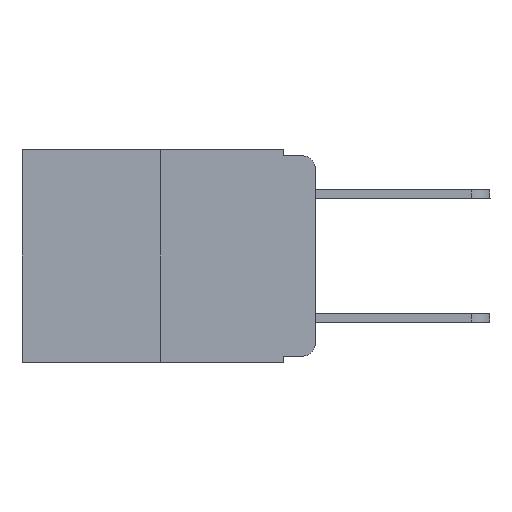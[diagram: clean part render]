
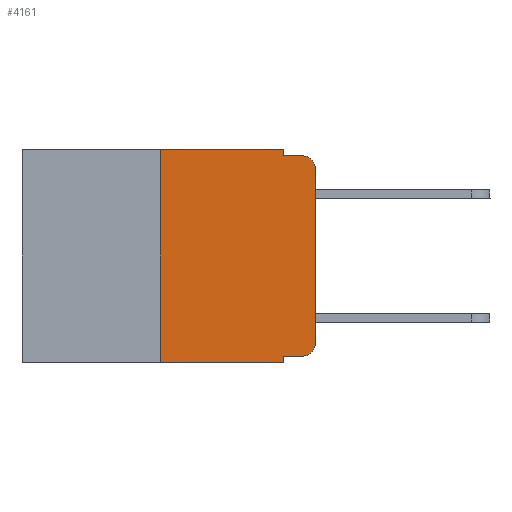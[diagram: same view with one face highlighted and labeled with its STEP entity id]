
A CAD part, left-side view. The second image highlights one B-rep face of the part: STEP entity #4161.
In plain terms, the highlighted planar face has unit normal (-1, 0, 0).
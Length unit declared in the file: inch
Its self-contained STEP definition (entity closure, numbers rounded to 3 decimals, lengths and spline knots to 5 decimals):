
#337 = EDGE_CURVE ( 'NONE', #19525, #14677, #18125, .T. ) ;
#1096 = DIRECTION ( 'NONE',  ( 0., 0., 1. ) ) ;
#1209 = EDGE_CURVE ( 'NONE', #7243, #7101, #4315, .T. ) ;
#1236 = CARTESIAN_POINT ( 'NONE',  ( 0., 0., -0.313 ) ) ;
#1493 = CARTESIAN_POINT ( 'NONE',  ( 0., 0.25, 0. ) ) ;
#1759 = VECTOR ( 'NONE', #14645, 39.37008 ) ;
#1848 = CARTESIAN_POINT ( 'NONE',  ( 0., 0.02, -0.313 ) ) ;
#2387 = CARTESIAN_POINT ( 'NONE',  ( 0., 0.051, -0.343 ) ) ;
#2466 = VECTOR ( 'NONE', #3647, 39.37008 ) ;
#2527 = EDGE_CURVE ( 'NONE', #3661, #4597, #5722, .T. ) ;
#2531 = CARTESIAN_POINT ( 'NONE',  ( 0., 0.25, -0.343 ) ) ;
#2651 = AXIS2_PLACEMENT_3D ( 'NONE', #13378, #22353, #20773 ) ;
#2685 = ORIENTED_EDGE ( 'NONE', *, *, #13599, .T. ) ;
#2820 = EDGE_CURVE ( 'NONE', #5294, #3661, #14529, .T. ) ;
#2821 = LINE ( 'NONE', #6984, #9242 ) ;
#3045 = VECTOR ( 'NONE', #20054, 39.37008 ) ;
#3330 = VERTEX_POINT ( 'NONE', #19326 ) ;
#3530 = CARTESIAN_POINT ( 'NONE',  ( 0., 0.473, 0. ) ) ;
#3574 = VECTOR ( 'NONE', #1096, 39.37008 ) ;
#3647 = DIRECTION ( 'NONE',  ( 0., -1., 0. ) ) ;
#3661 = VERTEX_POINT ( 'NONE', #1236 ) ;
#3689 = EDGE_CURVE ( 'NONE', #4597, #7101, #16062, .T. ) ;
#4014 = DIRECTION ( 'NONE',  ( 0., 0., 1. ) ) ;
#4109 = ORIENTED_EDGE ( 'NONE', *, *, #2820, .T. ) ;
#4161 = ADVANCED_FACE ( 'NONE', ( #6431 ), #8364, .F. ) ;
#4315 = LINE ( 'NONE', #7714, #1759 ) ;
#4552 = EDGE_CURVE ( 'NONE', #7382, #14677, #8307, .T. ) ;
#4597 = VERTEX_POINT ( 'NONE', #4881 ) ;
#4702 = ORIENTED_EDGE ( 'NONE', *, *, #12470, .F. ) ;
#4881 = CARTESIAN_POINT ( 'NONE',  ( 0., 0., -0.03 ) ) ;
#5246 = DIRECTION ( 'NONE',  ( -1., 0., 0. ) ) ;
#5294 = VERTEX_POINT ( 'NONE', #6202 ) ;
#5387 = DIRECTION ( 'NONE',  ( 0., 0., -1. ) ) ;
#5572 = ORIENTED_EDGE ( 'NONE', *, *, #337, .F. ) ;
#5597 = CARTESIAN_POINT ( 'NONE',  ( 0., 0.051, -0.01 ) ) ;
#5722 = LINE ( 'NONE', #7653, #15242 ) ;
#6202 = CARTESIAN_POINT ( 'NONE',  ( 0., 0.02, -0.333 ) ) ;
#6431 = FACE_OUTER_BOUND ( 'NONE', #11149, .T. ) ;
#6745 = CARTESIAN_POINT ( 'NONE',  ( 0., 0.02, -0.01 ) ) ;
#6984 = CARTESIAN_POINT ( 'NONE',  ( 0., 0.051, -0.333 ) ) ;
#7039 = DIRECTION ( 'NONE',  ( 0., -1., 0. ) ) ;
#7101 = VERTEX_POINT ( 'NONE', #6745 ) ;
#7243 = VERTEX_POINT ( 'NONE', #5597 ) ;
#7382 = VERTEX_POINT ( 'NONE', #2531 ) ;
#7636 = EDGE_CURVE ( 'NONE', #14393, #3330, #19115, .T. ) ;
#7653 = CARTESIAN_POINT ( 'NONE',  ( 0., 0., 0. ) ) ;
#7714 = CARTESIAN_POINT ( 'NONE',  ( 0., 0.051, -0.01 ) ) ;
#8109 = EDGE_CURVE ( 'NONE', #7382, #14393, #18479, .T. ) ;
#8254 = DIRECTION ( 'NONE',  ( 1., 0., 0. ) ) ;
#8307 = LINE ( 'NONE', #18985, #15568 ) ;
#8364 = PLANE ( 'NONE',  #16887 ) ;
#8692 = DIRECTION ( 'NONE',  ( 0., -1., 0. ) ) ;
#8924 = ORIENTED_EDGE ( 'NONE', *, *, #2527, .T. ) ;
#9170 = ORIENTED_EDGE ( 'NONE', *, *, #8109, .F. ) ;
#9242 = VECTOR ( 'NONE', #8692, 39.37008 ) ;
#10717 = ORIENTED_EDGE ( 'NONE', *, *, #1209, .F. ) ;
#11149 = EDGE_LOOP ( 'NONE', ( #8924, #22386, #10717, #4702, #20931, #9170, #12862, #5572, #2685, #4109 ) ) ;
#12470 = EDGE_CURVE ( 'NONE', #3330, #7243, #15722, .T. ) ;
#12862 = ORIENTED_EDGE ( 'NONE', *, *, #4552, .T. ) ;
#13378 = CARTESIAN_POINT ( 'NONE',  ( 0., 0.02, -0.03 ) ) ;
#13599 = EDGE_CURVE ( 'NONE', #19525, #5294, #2821, .T. ) ;
#13878 = DIRECTION ( 'NONE',  ( 0., 0., -1. ) ) ;
#14171 = AXIS2_PLACEMENT_3D ( 'NONE', #1848, #5246, #13878 ) ;
#14393 = VERTEX_POINT ( 'NONE', #1493 ) ;
#14529 = CIRCLE ( 'NONE', #14171, 0.02 ) ;
#14645 = DIRECTION ( 'NONE',  ( 0., -1., 0. ) ) ;
#14677 = VERTEX_POINT ( 'NONE', #2387 ) ;
#15242 = VECTOR ( 'NONE', #4014, 39.37008 ) ;
#15568 = VECTOR ( 'NONE', #7039, 39.37008 ) ;
#15722 = LINE ( 'NONE', #20964, #20460 ) ;
#16062 = CIRCLE ( 'NONE', #2651, 0.02 ) ;
#16887 = AXIS2_PLACEMENT_3D ( 'NONE', #18930, #8254, #20301 ) ;
#18125 = LINE ( 'NONE', #21635, #3045 ) ;
#18479 = LINE ( 'NONE', #19957, #3574 ) ;
#18930 = CARTESIAN_POINT ( 'NONE',  ( 0., 0.473, 0. ) ) ;
#18985 = CARTESIAN_POINT ( 'NONE',  ( 0., 0.473, -0.343 ) ) ;
#19115 = LINE ( 'NONE', #3530, #2466 ) ;
#19326 = CARTESIAN_POINT ( 'NONE',  ( 0., 0.051, 0. ) ) ;
#19525 = VERTEX_POINT ( 'NONE', #21820 ) ;
#19957 = CARTESIAN_POINT ( 'NONE',  ( 0., 0.25, 0. ) ) ;
#20054 = DIRECTION ( 'NONE',  ( 0., 0., -1. ) ) ;
#20301 = DIRECTION ( 'NONE',  ( 0., 0., -1. ) ) ;
#20460 = VECTOR ( 'NONE', #5387, 39.37008 ) ;
#20773 = DIRECTION ( 'NONE',  ( 0., 0., -1. ) ) ;
#20931 = ORIENTED_EDGE ( 'NONE', *, *, #7636, .F. ) ;
#20964 = CARTESIAN_POINT ( 'NONE',  ( 0., 0.051, 0. ) ) ;
#21635 = CARTESIAN_POINT ( 'NONE',  ( 0., 0.051, 0. ) ) ;
#21820 = CARTESIAN_POINT ( 'NONE',  ( 0., 0.051, -0.333 ) ) ;
#22353 = DIRECTION ( 'NONE',  ( -1., 0., 0. ) ) ;
#22386 = ORIENTED_EDGE ( 'NONE', *, *, #3689, .T. ) ;
